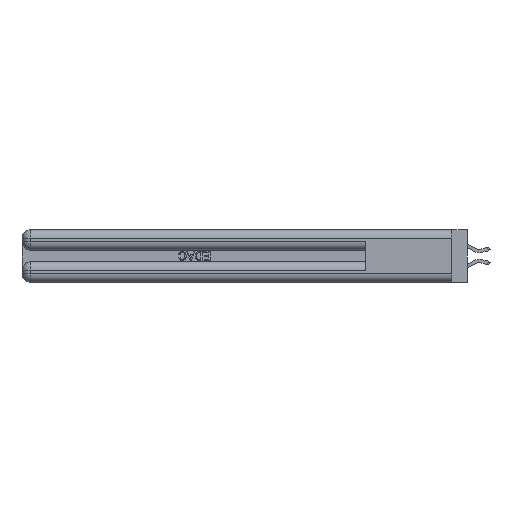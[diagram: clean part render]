
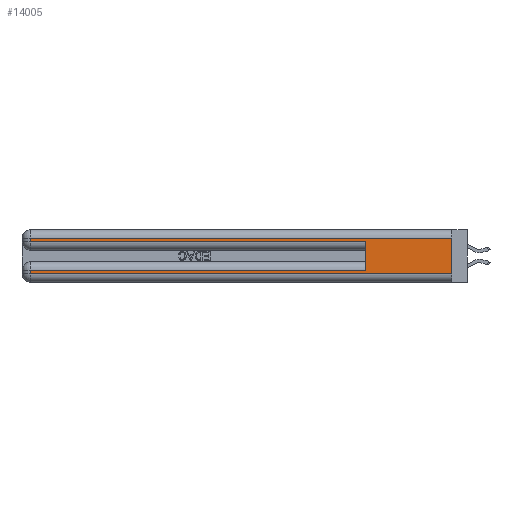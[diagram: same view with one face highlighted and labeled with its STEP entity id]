
A CAD part, left-side view. The second image highlights one B-rep face of the part: STEP entity #14005.
In plain terms, the highlighted planar face has unit normal (-1, 0, 0).
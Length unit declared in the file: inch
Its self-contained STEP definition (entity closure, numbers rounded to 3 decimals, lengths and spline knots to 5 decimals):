
#1040 = CARTESIAN_POINT ( 'NONE',  ( 0., 0., 0.085 ) ) ;
#1395 = VERTEX_POINT ( 'NONE', #21570 ) ;
#3991 = DIRECTION ( 'NONE',  ( 0., 0., -1. ) ) ;
#6028 = DIRECTION ( 'NONE',  ( 0., 1., 0. ) ) ;
#7169 = VERTEX_POINT ( 'NONE', #35106 ) ;
#8353 = CARTESIAN_POINT ( 'NONE',  ( 0., 0.6, 0.085 ) ) ;
#8776 = CARTESIAN_POINT ( 'NONE',  ( 0., 0.6, 0.145 ) ) ;
#8930 = CARTESIAN_POINT ( 'NONE',  ( 0., 2.94, 0.31 ) ) ;
#10480 = EDGE_CURVE ( 'NONE', #37464, #17831, #23505, .T. ) ;
#10765 = VECTOR ( 'NONE', #16864, 39.37008 ) ;
#10779 = CARTESIAN_POINT ( 'NONE',  ( 0., 2.94, 0.37 ) ) ;
#11335 = ORIENTED_EDGE ( 'NONE', *, *, #14505, .F. ) ;
#12615 = CARTESIAN_POINT ( 'NONE',  ( 0., 2.94, 0.285 ) ) ;
#12674 = VECTOR ( 'NONE', #12958, 39.37008 ) ;
#12958 = DIRECTION ( 'NONE',  ( 0., -1., 0. ) ) ;
#13098 = CARTESIAN_POINT ( 'NONE',  ( 0., 0., 0.37 ) ) ;
#13411 = DIRECTION ( 'NONE',  ( 1., 0., 0. ) ) ;
#14005 = ADVANCED_FACE ( 'NONE', ( #41998 ), #35089, .F. ) ;
#14067 = CARTESIAN_POINT ( 'NONE',  ( 0., 0., 0.31 ) ) ;
#14079 = LINE ( 'NONE', #1040, #45820 ) ;
#14492 = VERTEX_POINT ( 'NONE', #23240 ) ;
#14505 = EDGE_CURVE ( 'NONE', #25716, #7169, #20379, .T. ) ;
#16864 = DIRECTION ( 'NONE',  ( 0., 0., -1. ) ) ;
#17831 = VERTEX_POINT ( 'NONE', #12615 ) ;
#17893 = LINE ( 'NONE', #10779, #38340 ) ;
#18621 = EDGE_CURVE ( 'NONE', #14492, #1395, #17893, .T. ) ;
#19454 = EDGE_CURVE ( 'NONE', #25716, #37464, #43972, .T. ) ;
#20239 = ORIENTED_EDGE ( 'NONE', *, *, #34195, .T. ) ;
#20379 = LINE ( 'NONE', #38734, #10765 ) ;
#21398 = CARTESIAN_POINT ( 'NONE',  ( 0., 0.6, 0.285 ) ) ;
#21570 = CARTESIAN_POINT ( 'NONE',  ( 0., 2.94, 0.06 ) ) ;
#23220 = DIRECTION ( 'NONE',  ( 0., 0., 1. ) ) ;
#23240 = CARTESIAN_POINT ( 'NONE',  ( 0., 2.94, 0.085 ) ) ;
#23505 = LINE ( 'NONE', #41967, #42751 ) ;
#25391 = AXIS2_PLACEMENT_3D ( 'NONE', #13098, #13411, #27666 ) ;
#25480 = ORIENTED_EDGE ( 'NONE', *, *, #19454, .T. ) ;
#25716 = VERTEX_POINT ( 'NONE', #14067 ) ;
#27566 = DIRECTION ( 'NONE',  ( 0., 0., -1. ) ) ;
#27666 = DIRECTION ( 'NONE',  ( 0., 0., -1. ) ) ;
#29151 = VERTEX_POINT ( 'NONE', #8353 ) ;
#29193 = EDGE_LOOP ( 'NONE', ( #11335, #25480, #31771, #40205, #33530, #20239, #33336, #34997 ) ) ;
#30648 = DIRECTION ( 'NONE',  ( 0., 1., 0. ) ) ;
#30939 = VECTOR ( 'NONE', #6028, 39.37008 ) ;
#31771 = ORIENTED_EDGE ( 'NONE', *, *, #10480, .T. ) ;
#32516 = VERTEX_POINT ( 'NONE', #21398 ) ;
#33336 = ORIENTED_EDGE ( 'NONE', *, *, #18621, .T. ) ;
#33530 = ORIENTED_EDGE ( 'NONE', *, *, #37518, .F. ) ;
#34195 = EDGE_CURVE ( 'NONE', #29151, #14492, #14079, .T. ) ;
#34997 = ORIENTED_EDGE ( 'NONE', *, *, #36959, .T. ) ;
#35082 = CARTESIAN_POINT ( 'NONE',  ( 0., 0., 0.31 ) ) ;
#35089 = PLANE ( 'NONE',  #25391 ) ;
#35106 = CARTESIAN_POINT ( 'NONE',  ( 0., 0., 0.06 ) ) ;
#35872 = EDGE_CURVE ( 'NONE', #17831, #32516, #37103, .T. ) ;
#36153 = DIRECTION ( 'NONE',  ( 0., -1., 0. ) ) ;
#36959 = EDGE_CURVE ( 'NONE', #1395, #7169, #40416, .T. ) ;
#37103 = LINE ( 'NONE', #38867, #40505 ) ;
#37464 = VERTEX_POINT ( 'NONE', #8930 ) ;
#37518 = EDGE_CURVE ( 'NONE', #29151, #32516, #45501, .T. ) ;
#38340 = VECTOR ( 'NONE', #3991, 39.37008 ) ;
#38734 = CARTESIAN_POINT ( 'NONE',  ( 0., 0., 0.37 ) ) ;
#38867 = CARTESIAN_POINT ( 'NONE',  ( 0., 0., 0.285 ) ) ;
#40205 = ORIENTED_EDGE ( 'NONE', *, *, #35872, .T. ) ;
#40416 = LINE ( 'NONE', #42088, #12674 ) ;
#40505 = VECTOR ( 'NONE', #36153, 39.37008 ) ;
#41967 = CARTESIAN_POINT ( 'NONE',  ( 0., 2.94, 0.37 ) ) ;
#41998 = FACE_OUTER_BOUND ( 'NONE', #29193, .T. ) ;
#42088 = CARTESIAN_POINT ( 'NONE',  ( 0., 0., 0.06 ) ) ;
#42751 = VECTOR ( 'NONE', #27566, 39.37008 ) ;
#43775 = VECTOR ( 'NONE', #23220, 39.37008 ) ;
#43972 = LINE ( 'NONE', #35082, #30939 ) ;
#45501 = LINE ( 'NONE', #8776, #43775 ) ;
#45820 = VECTOR ( 'NONE', #30648, 39.37008 ) ;
